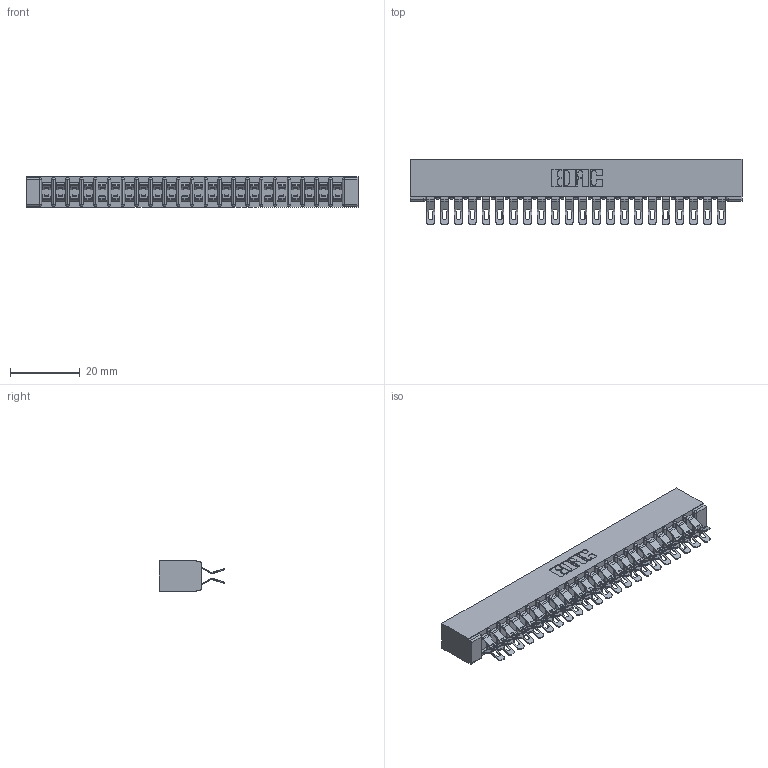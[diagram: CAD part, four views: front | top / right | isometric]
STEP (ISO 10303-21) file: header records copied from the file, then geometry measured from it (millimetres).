
FILE_DESCRIPTION (( 'STEP AP203' ), '1' );
FILE_NAME ('357-044-555-201.STEP', '2019-09-18T07:36:37', ( '' ), ( '' ), 'SwSTEP 2.0', 'SolidWorks 2016', '' );
FILE_SCHEMA (( 'CONFIG_CONTROL_DESIGN' ));
Length unit declared in the file: inch
Products named in the file (3): 307-290-001_555; 307 Part_No Mounting Lugs; 357-044-555-201
Assembly tree (45 placements, depth 2):
  357-044-555-201
    307 Part_No Mounting Lugs
    307-290-001_555  x44
Bounding box: 95.05 x 18.75 x 8.71 mm (x, y, z)
Volume: 6581.3 mm3; surface area: 12818.9 mm2
Topology: 45 solids, 45 shells, 2817 faces, 8263 edges, 5386 vertices
Faces by surface type: plane 1562, cylinder 1209, sphere 46
Entity records: 22289 total; most frequent: CARTESIAN_POINT 3654, ORIENTED_EDGE 3620, DIRECTION 3594, EDGE_CURVE 1810, VECTOR 1370, LINE 1370, VERTEX_POINT 1172, AXIS2_PLACEMENT_3D 1112
